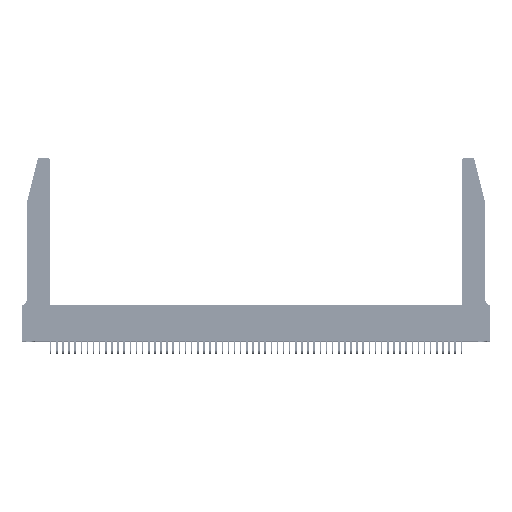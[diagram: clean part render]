
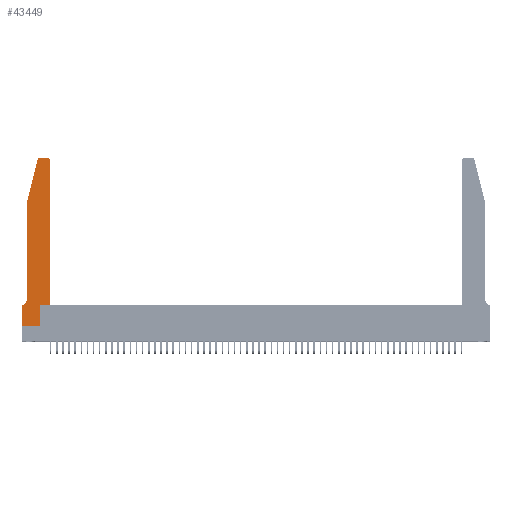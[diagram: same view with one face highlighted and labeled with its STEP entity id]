
A CAD part, top view. The second image highlights one B-rep face of the part: STEP entity #43449.
In plain terms, the highlighted planar face has unit normal (0, 0, 1).
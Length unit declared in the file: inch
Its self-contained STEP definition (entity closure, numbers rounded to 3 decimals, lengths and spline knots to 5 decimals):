
#1133 = EDGE_CURVE ( 'NONE', #4631, #20793, #50221, .T. ) ;
#2829 = LINE ( 'NONE', #46798, #13077 ) ;
#3600 = CARTESIAN_POINT ( 'NONE',  ( 0.4505, 0.35, 0.37 ) ) ;
#4631 = VERTEX_POINT ( 'NONE', #52314 ) ;
#5227 = CARTESIAN_POINT ( 'NONE',  ( 0.0755, 2., 0.37 ) ) ;
#5277 = VECTOR ( 'NONE', #48576, 39.37008 ) ;
#5647 = LINE ( 'NONE', #48672, #27549 ) ;
#5694 = EDGE_LOOP ( 'NONE', ( #50773, #20109, #27413, #54516, #23534, #40198, #50181, #11986, #35045, #14141, #16805, #7397 ) ) ;
#5927 = CIRCLE ( 'NONE', #18380, 0.03 ) ;
#7245 = EDGE_CURVE ( 'NONE', #27093, #31685, #34787, .T. ) ;
#7397 = ORIENTED_EDGE ( 'NONE', *, *, #16577, .T. ) ;
#7573 = PLANE ( 'NONE',  #53949 ) ;
#7774 = EDGE_CURVE ( 'NONE', #20793, #12616, #29309, .T. ) ;
#8736 = EDGE_CURVE ( 'NONE', #16596, #56164, #18326, .T. ) ;
#9914 = FACE_OUTER_BOUND ( 'NONE', #5694, .T. ) ;
#10099 = CARTESIAN_POINT ( 'NONE',  ( 0.0055, 0.42, 0.37 ) ) ;
#11961 = DIRECTION ( 'NONE',  ( 1., 0., 0. ) ) ;
#11986 = ORIENTED_EDGE ( 'NONE', *, *, #19087, .T. ) ;
#12158 = CARTESIAN_POINT ( 'NONE',  ( 0.25487, 2.72718, 0.37 ) ) ;
#12330 = LINE ( 'NONE', #24546, #55738 ) ;
#12558 = VERTEX_POINT ( 'NONE', #51482 ) ;
#12616 = VERTEX_POINT ( 'NONE', #47508 ) ;
#13077 = VECTOR ( 'NONE', #20845, 39.37008 ) ;
#13746 = CARTESIAN_POINT ( 'NONE',  ( 0.4505, 0.35, 0.37 ) ) ;
#14141 = ORIENTED_EDGE ( 'NONE', *, *, #1133, .T. ) ;
#14513 = DIRECTION ( 'NONE',  ( -1., 0., 0. ) ) ;
#15054 = EDGE_CURVE ( 'NONE', #31685, #41162, #2829, .T. ) ;
#15633 = VECTOR ( 'NONE', #35527, 39.37008 ) ;
#16206 = CARTESIAN_POINT ( 'NONE',  ( 0., 0.35, 0.37 ) ) ;
#16577 = EDGE_CURVE ( 'NONE', #12616, #44953, #53255, .T. ) ;
#16596 = VERTEX_POINT ( 'NONE', #12158 ) ;
#16805 = ORIENTED_EDGE ( 'NONE', *, *, #7774, .T. ) ;
#16932 = EDGE_CURVE ( 'NONE', #56164, #19922, #27642, .T. ) ;
#17243 = VERTEX_POINT ( 'NONE', #29362 ) ;
#17616 = DIRECTION ( 'NONE',  ( 0., 0., 1. ) ) ;
#18326 = LINE ( 'NONE', #5227, #5277 ) ;
#18380 = AXIS2_PLACEMENT_3D ( 'NONE', #43635, #17616, #47938 ) ;
#19087 = EDGE_CURVE ( 'NONE', #41162, #12558, #12330, .T. ) ;
#19922 = VERTEX_POINT ( 'NONE', #51677 ) ;
#20109 = ORIENTED_EDGE ( 'NONE', *, *, #42598, .T. ) ;
#20390 = VECTOR ( 'NONE', #53810, 39.37008 ) ;
#20779 = CARTESIAN_POINT ( 'NONE',  ( 0.4205, 2.72, 0.37 ) ) ;
#20793 = VERTEX_POINT ( 'NONE', #31456 ) ;
#20845 = DIRECTION ( 'NONE',  ( 0., -1., 0. ) ) ;
#20930 = CARTESIAN_POINT ( 'NONE',  ( 0.0055, 0.35, 0.37 ) ) ;
#23279 = CIRCLE ( 'NONE', #46109, 0.07 ) ;
#23534 = ORIENTED_EDGE ( 'NONE', *, *, #47005, .T. ) ;
#23764 = CARTESIAN_POINT ( 'NONE',  ( 0.2865, 0.35, 0.37 ) ) ;
#24546 = CARTESIAN_POINT ( 'NONE',  ( 0., 0., 0.37 ) ) ;
#25159 = DIRECTION ( 'NONE',  ( 1., 0., 0. ) ) ;
#27093 = VERTEX_POINT ( 'NONE', #20930 ) ;
#27413 = ORIENTED_EDGE ( 'NONE', *, *, #8736, .T. ) ;
#27425 = CARTESIAN_POINT ( 'NONE',  ( 0., 0.35, 0.37 ) ) ;
#27438 = DIRECTION ( 'NONE',  ( 0., -1., 0. ) ) ;
#27509 = CARTESIAN_POINT ( 'NONE',  ( 0.4205, 2.75, 0.37 ) ) ;
#27549 = VECTOR ( 'NONE', #35710, 39.37008 ) ;
#27642 = LINE ( 'NONE', #52935, #47904 ) ;
#27905 = VECTOR ( 'NONE', #42882, 39.37008 ) ;
#29309 = LINE ( 'NONE', #3600, #27905 ) ;
#29362 = CARTESIAN_POINT ( 'NONE',  ( 0.284, 2.75, 0.37 ) ) ;
#30669 = LINE ( 'NONE', #23764, #20390 ) ;
#31456 = CARTESIAN_POINT ( 'NONE',  ( 0.4505, 0.35, 0.37 ) ) ;
#31685 = VERTEX_POINT ( 'NONE', #27425 ) ;
#31720 = DIRECTION ( 'NONE',  ( -1., 0., 0. ) ) ;
#33349 = DIRECTION ( 'NONE',  ( 1., 0., 0. ) ) ;
#34787 = LINE ( 'NONE', #40393, #54967 ) ;
#35045 = ORIENTED_EDGE ( 'NONE', *, *, #54891, .T. ) ;
#35527 = DIRECTION ( 'NONE',  ( 1., 0., 0. ) ) ;
#35710 = DIRECTION ( 'NONE',  ( -1., 0., 0. ) ) ;
#38099 = DIRECTION ( 'NONE',  ( 0., 0., 1. ) ) ;
#39762 = AXIS2_PLACEMENT_3D ( 'NONE', #20779, #51071, #25159 ) ;
#40198 = ORIENTED_EDGE ( 'NONE', *, *, #7245, .T. ) ;
#40393 = CARTESIAN_POINT ( 'NONE',  ( 0.0755, 0.35, 0.37 ) ) ;
#40595 = DIRECTION ( 'NONE',  ( 0., 0., -1. ) ) ;
#41162 = VERTEX_POINT ( 'NONE', #42461 ) ;
#42461 = CARTESIAN_POINT ( 'NONE',  ( 0., 0., 0.37 ) ) ;
#42598 = EDGE_CURVE ( 'NONE', #17243, #16596, #5927, .T. ) ;
#42882 = DIRECTION ( 'NONE',  ( 0., 1., 0. ) ) ;
#43449 = ADVANCED_FACE ( 'NONE', ( #9914 ), #7573, .T. ) ;
#43635 = CARTESIAN_POINT ( 'NONE',  ( 0.284, 2.72, 0.37 ) ) ;
#44897 = EDGE_CURVE ( 'NONE', #44953, #17243, #5647, .T. ) ;
#44953 = VERTEX_POINT ( 'NONE', #27509 ) ;
#46109 = AXIS2_PLACEMENT_3D ( 'NONE', #10099, #40595, #14513 ) ;
#46798 = CARTESIAN_POINT ( 'NONE',  ( 0., 0., 0.37 ) ) ;
#47005 = EDGE_CURVE ( 'NONE', #19922, #27093, #23279, .T. ) ;
#47508 = CARTESIAN_POINT ( 'NONE',  ( 0.4505, 2.72, 0.37 ) ) ;
#47904 = VECTOR ( 'NONE', #27438, 39.37008 ) ;
#47938 = DIRECTION ( 'NONE',  ( 1., 0., 0. ) ) ;
#48576 = DIRECTION ( 'NONE',  ( -0.239, -0.971, 0. ) ) ;
#48672 = CARTESIAN_POINT ( 'NONE',  ( 0.2605, 2.75, 0.37 ) ) ;
#50181 = ORIENTED_EDGE ( 'NONE', *, *, #15054, .T. ) ;
#50221 = LINE ( 'NONE', #13746, #15633 ) ;
#50773 = ORIENTED_EDGE ( 'NONE', *, *, #44897, .T. ) ;
#51071 = DIRECTION ( 'NONE',  ( 0., 0., 1. ) ) ;
#51482 = CARTESIAN_POINT ( 'NONE',  ( 0.2865, 0., 0.37 ) ) ;
#51677 = CARTESIAN_POINT ( 'NONE',  ( 0.0755, 0.42, 0.37 ) ) ;
#52314 = CARTESIAN_POINT ( 'NONE',  ( 0.2865, 0.35, 0.37 ) ) ;
#52467 = CARTESIAN_POINT ( 'NONE',  ( 0.0755, 2., 0.37 ) ) ;
#52935 = CARTESIAN_POINT ( 'NONE',  ( 0.0755, 2., 0.37 ) ) ;
#53255 = CIRCLE ( 'NONE', #39762, 0.03 ) ;
#53810 = DIRECTION ( 'NONE',  ( 0., 1., 0. ) ) ;
#53949 = AXIS2_PLACEMENT_3D ( 'NONE', #16206, #38099, #11961 ) ;
#54516 = ORIENTED_EDGE ( 'NONE', *, *, #16932, .T. ) ;
#54891 = EDGE_CURVE ( 'NONE', #12558, #4631, #30669, .T. ) ;
#54967 = VECTOR ( 'NONE', #31720, 39.37008 ) ;
#55738 = VECTOR ( 'NONE', #33349, 39.37008 ) ;
#56164 = VERTEX_POINT ( 'NONE', #52467 ) ;
